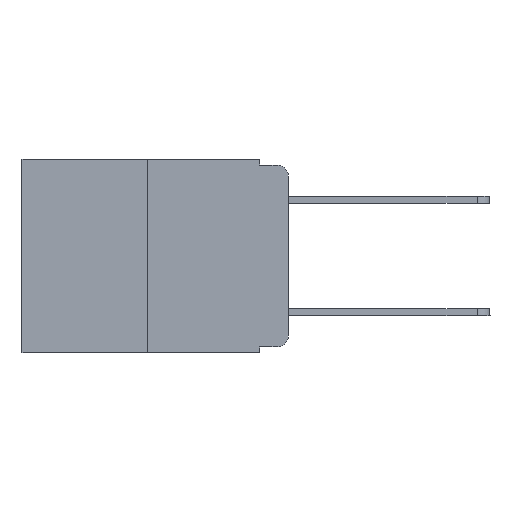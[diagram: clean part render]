
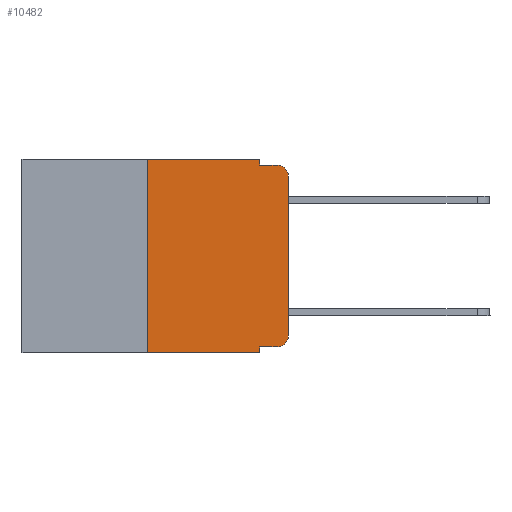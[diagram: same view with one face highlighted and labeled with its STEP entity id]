
A CAD part, left-side view. The second image highlights one B-rep face of the part: STEP entity #10482.
In plain terms, the highlighted planar face has unit normal (-1, 0, 0).
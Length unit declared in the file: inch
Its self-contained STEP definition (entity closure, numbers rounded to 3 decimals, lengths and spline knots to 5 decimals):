
#465 = EDGE_CURVE ( 'NONE', #9099, #16869, #15934, .T. ) ;
#628 = EDGE_CURVE ( 'NONE', #2871, #2681, #1880, .T. ) ;
#996 = AXIS2_PLACEMENT_3D ( 'NONE', #10161, #19075, #12952 ) ;
#1095 = DIRECTION ( 'NONE',  ( 0., 0., -1. ) ) ;
#1135 = DIRECTION ( 'NONE',  ( 0., 0., -1. ) ) ;
#1201 = ORIENTED_EDGE ( 'NONE', *, *, #13139, .F. ) ;
#1327 = ORIENTED_EDGE ( 'NONE', *, *, #8347, .T. ) ;
#1449 = EDGE_LOOP ( 'NONE', ( #1327, #4392, #4620, #1201, #5908, #11030, #7488, #8033, #6290, #10055 ) ) ;
#1563 = CIRCLE ( 'NONE', #18480, 0.02 ) ;
#1880 = LINE ( 'NONE', #19255, #8816 ) ;
#1973 = VECTOR ( 'NONE', #18676, 39.37008 ) ;
#2036 = CARTESIAN_POINT ( 'NONE',  ( 0., 0.02, -0.03 ) ) ;
#2037 = CARTESIAN_POINT ( 'NONE',  ( 0., 0.25, -0.343 ) ) ;
#2235 = VECTOR ( 'NONE', #9015, 39.37008 ) ;
#2311 = LINE ( 'NONE', #7648, #14464 ) ;
#2681 = VERTEX_POINT ( 'NONE', #15448 ) ;
#2871 = VERTEX_POINT ( 'NONE', #4741 ) ;
#3396 = DIRECTION ( 'NONE',  ( 0., -1., 0. ) ) ;
#3654 = VERTEX_POINT ( 'NONE', #5731 ) ;
#3918 = DIRECTION ( 'NONE',  ( 0., -1., 0. ) ) ;
#4392 = ORIENTED_EDGE ( 'NONE', *, *, #16805, .T. ) ;
#4616 = FACE_OUTER_BOUND ( 'NONE', #1449, .T. ) ;
#4620 = ORIENTED_EDGE ( 'NONE', *, *, #10249, .F. ) ;
#4741 = CARTESIAN_POINT ( 'NONE',  ( 0., 0.051, -0.333 ) ) ;
#4791 = DIRECTION ( 'NONE',  ( 0., 0., -1. ) ) ;
#4872 = VERTEX_POINT ( 'NONE', #10875 ) ;
#4906 = VECTOR ( 'NONE', #3396, 39.37008 ) ;
#5343 = LINE ( 'NONE', #13956, #2235 ) ;
#5510 = CARTESIAN_POINT ( 'NONE',  ( 0., 0.051, 0. ) ) ;
#5540 = LINE ( 'NONE', #5510, #13158 ) ;
#5731 = CARTESIAN_POINT ( 'NONE',  ( 0., 0.051, 0. ) ) ;
#5908 = ORIENTED_EDGE ( 'NONE', *, *, #17598, .F. ) ;
#6290 = ORIENTED_EDGE ( 'NONE', *, *, #628, .T. ) ;
#6936 = VERTEX_POINT ( 'NONE', #11522 ) ;
#7488 = ORIENTED_EDGE ( 'NONE', *, *, #465, .T. ) ;
#7648 = CARTESIAN_POINT ( 'NONE',  ( 0., 0., 0. ) ) ;
#7821 = LINE ( 'NONE', #12585, #11405 ) ;
#7879 = EDGE_CURVE ( 'NONE', #2871, #16869, #7821, .T. ) ;
#8033 = ORIENTED_EDGE ( 'NONE', *, *, #7879, .F. ) ;
#8347 = EDGE_CURVE ( 'NONE', #4872, #6936, #2311, .T. ) ;
#8497 = CARTESIAN_POINT ( 'NONE',  ( 0., 0.02, -0.01 ) ) ;
#8816 = VECTOR ( 'NONE', #3918, 39.37008 ) ;
#8838 = CARTESIAN_POINT ( 'NONE',  ( 0., 0.25, 0. ) ) ;
#9015 = DIRECTION ( 'NONE',  ( 0., -1., 0. ) ) ;
#9099 = VERTEX_POINT ( 'NONE', #2037 ) ;
#9289 = VECTOR ( 'NONE', #9424, 39.37008 ) ;
#9424 = DIRECTION ( 'NONE',  ( 0., -1., 0. ) ) ;
#9486 = CARTESIAN_POINT ( 'NONE',  ( 0., 0.25, 0. ) ) ;
#10055 = ORIENTED_EDGE ( 'NONE', *, *, #17797, .T. ) ;
#10161 = CARTESIAN_POINT ( 'NONE',  ( 0., 0.02, -0.313 ) ) ;
#10249 = EDGE_CURVE ( 'NONE', #11618, #14385, #5343, .T. ) ;
#10470 = PLANE ( 'NONE',  #15314 ) ;
#10482 = ADVANCED_FACE ( 'NONE', ( #4616 ), #10470, .F. ) ;
#10778 = DIRECTION ( 'NONE',  ( 0., 0., 1. ) ) ;
#10875 = CARTESIAN_POINT ( 'NONE',  ( 0., 0., -0.313 ) ) ;
#10894 = CARTESIAN_POINT ( 'NONE',  ( 0., 0.473, -0.343 ) ) ;
#11030 = ORIENTED_EDGE ( 'NONE', *, *, #12554, .F. ) ;
#11146 = LINE ( 'NONE', #14040, #4906 ) ;
#11405 = VECTOR ( 'NONE', #4791, 39.37008 ) ;
#11522 = CARTESIAN_POINT ( 'NONE',  ( 0., 0., -0.03 ) ) ;
#11618 = VERTEX_POINT ( 'NONE', #13984 ) ;
#12020 = DIRECTION ( 'NONE',  ( 1., 0., 0. ) ) ;
#12554 = EDGE_CURVE ( 'NONE', #9099, #14562, #19136, .T. ) ;
#12585 = CARTESIAN_POINT ( 'NONE',  ( 0., 0.051, 0. ) ) ;
#12692 = DIRECTION ( 'NONE',  ( -1., 0., 0. ) ) ;
#12952 = DIRECTION ( 'NONE',  ( 0., 0., -1. ) ) ;
#13139 = EDGE_CURVE ( 'NONE', #3654, #11618, #5540, .T. ) ;
#13158 = VECTOR ( 'NONE', #1095, 39.37008 ) ;
#13538 = CARTESIAN_POINT ( 'NONE',  ( 0., 0.473, 0. ) ) ;
#13956 = CARTESIAN_POINT ( 'NONE',  ( 0., 0.051, -0.01 ) ) ;
#13984 = CARTESIAN_POINT ( 'NONE',  ( 0., 0.051, -0.01 ) ) ;
#14040 = CARTESIAN_POINT ( 'NONE',  ( 0., 0.473, 0. ) ) ;
#14385 = VERTEX_POINT ( 'NONE', #8497 ) ;
#14464 = VECTOR ( 'NONE', #10778, 39.37008 ) ;
#14562 = VERTEX_POINT ( 'NONE', #8838 ) ;
#14686 = CARTESIAN_POINT ( 'NONE',  ( 0., 0.051, -0.343 ) ) ;
#15314 = AXIS2_PLACEMENT_3D ( 'NONE', #13538, #12020, #1135 ) ;
#15448 = CARTESIAN_POINT ( 'NONE',  ( 0., 0.02, -0.333 ) ) ;
#15934 = LINE ( 'NONE', #10894, #9289 ) ;
#16387 = CIRCLE ( 'NONE', #996, 0.02 ) ;
#16805 = EDGE_CURVE ( 'NONE', #6936, #14385, #1563, .T. ) ;
#16869 = VERTEX_POINT ( 'NONE', #14686 ) ;
#17598 = EDGE_CURVE ( 'NONE', #14562, #3654, #11146, .T. ) ;
#17745 = DIRECTION ( 'NONE',  ( 0., 0., -1. ) ) ;
#17797 = EDGE_CURVE ( 'NONE', #2681, #4872, #16387, .T. ) ;
#18480 = AXIS2_PLACEMENT_3D ( 'NONE', #2036, #12692, #17745 ) ;
#18676 = DIRECTION ( 'NONE',  ( 0., 0., 1. ) ) ;
#19075 = DIRECTION ( 'NONE',  ( -1., 0., 0. ) ) ;
#19136 = LINE ( 'NONE', #9486, #1973 ) ;
#19255 = CARTESIAN_POINT ( 'NONE',  ( 0., 0.051, -0.333 ) ) ;
